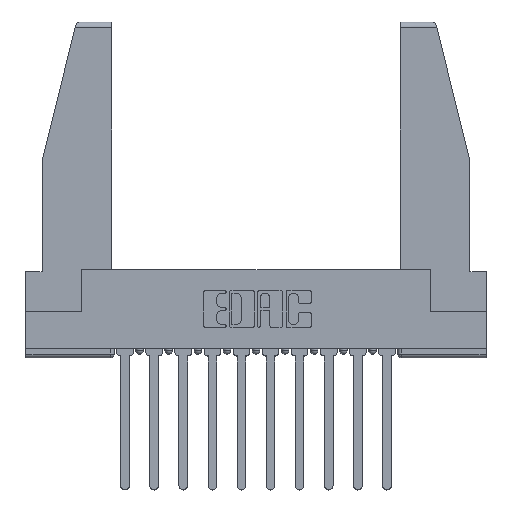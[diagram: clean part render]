
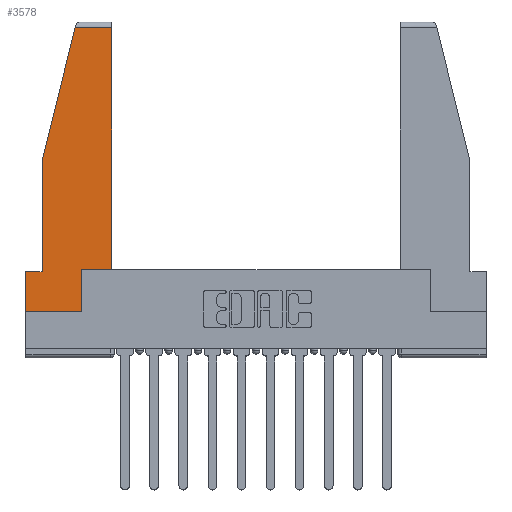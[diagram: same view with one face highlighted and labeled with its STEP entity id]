
A CAD part, top view. The second image highlights one B-rep face of the part: STEP entity #3578.
In plain terms, the highlighted planar face has unit normal (0, 0, 1).
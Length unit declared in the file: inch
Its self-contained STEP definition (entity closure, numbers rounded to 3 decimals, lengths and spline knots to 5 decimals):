
#171 = VECTOR ( 'NONE', #4945, 39.37008 ) ;
#489 = ORIENTED_EDGE ( 'NONE', *, *, #1004, .T. ) ;
#675 = LINE ( 'NONE', #2771, #14675 ) ;
#927 = FACE_OUTER_BOUND ( 'NONE', #11522, .T. ) ;
#1004 = EDGE_CURVE ( 'NONE', #10563, #9071, #10945, .T. ) ;
#1023 = CARTESIAN_POINT ( 'NONE',  ( 0.2636, 1.52, 0. ) ) ;
#1205 = EDGE_CURVE ( 'NONE', #8039, #13820, #3574, .T. ) ;
#1233 = VERTEX_POINT ( 'NONE', #8823 ) ;
#1274 = VECTOR ( 'NONE', #9186, 39.37008 ) ;
#1566 = EDGE_CURVE ( 'NONE', #1233, #8039, #10570, .T. ) ;
#1838 = DIRECTION ( 'NONE',  ( 0., 1., 0. ) ) ;
#2105 = VECTOR ( 'NONE', #6671, 39.37008 ) ;
#2409 = AXIS2_PLACEMENT_3D ( 'NONE', #7651, #11074, #8683 ) ;
#2624 = VERTEX_POINT ( 'NONE', #4546 ) ;
#2654 = ORIENTED_EDGE ( 'NONE', *, *, #11055, .T. ) ;
#2771 = CARTESIAN_POINT ( 'NONE',  ( 0., 0.21, 0. ) ) ;
#2823 = CARTESIAN_POINT ( 'NONE',  ( 0., 0.21, 0. ) ) ;
#2879 = DIRECTION ( 'NONE',  ( 0., -1., 0. ) ) ;
#3443 = EDGE_CURVE ( 'NONE', #7910, #9589, #12347, .T. ) ;
#3574 = LINE ( 'NONE', #14794, #12434 ) ;
#3578 = ADVANCED_FACE ( 'NONE', ( #927 ), #8742, .T. ) ;
#3805 = CARTESIAN_POINT ( 'NONE',  ( 0.461, 0.223, 0. ) ) ;
#4299 = VECTOR ( 'NONE', #13237, 39.37008 ) ;
#4369 = CARTESIAN_POINT ( 'NONE',  ( 0., 1.52, 0. ) ) ;
#4546 = CARTESIAN_POINT ( 'NONE',  ( 0.297, 0.223, 0. ) ) ;
#4945 = DIRECTION ( 'NONE',  ( 0., 1., 0. ) ) ;
#5190 = VECTOR ( 'NONE', #1838, 39.37008 ) ;
#5226 = CARTESIAN_POINT ( 'NONE',  ( 0.086, 0.21, 0. ) ) ;
#5296 = CARTESIAN_POINT ( 'NONE',  ( 0.297, 0., 0. ) ) ;
#5625 = VECTOR ( 'NONE', #13990, 39.37008 ) ;
#5702 = CARTESIAN_POINT ( 'NONE',  ( 0., 0., 0. ) ) ;
#6037 = CARTESIAN_POINT ( 'NONE',  ( 0.271, 1.55, 0. ) ) ;
#6671 = DIRECTION ( 'NONE',  ( 1., 0., 0. ) ) ;
#7025 = CARTESIAN_POINT ( 'NONE',  ( 0.461, 1.52, 0. ) ) ;
#7330 = CARTESIAN_POINT ( 'NONE',  ( 0.297, 0., 0. ) ) ;
#7535 = DIRECTION ( 'NONE',  ( 0., -1., 0. ) ) ;
#7651 = CARTESIAN_POINT ( 'NONE',  ( 0., 0., 0. ) ) ;
#7776 = CARTESIAN_POINT ( 'NONE',  ( 0., 0., 0. ) ) ;
#7782 = VERTEX_POINT ( 'NONE', #1023 ) ;
#7910 = VERTEX_POINT ( 'NONE', #8453 ) ;
#8039 = VERTEX_POINT ( 'NONE', #5226 ) ;
#8453 = CARTESIAN_POINT ( 'NONE',  ( 0.461, 0.223, 0. ) ) ;
#8683 = DIRECTION ( 'NONE',  ( 1., 0., 0. ) ) ;
#8742 = PLANE ( 'NONE',  #2409 ) ;
#8823 = CARTESIAN_POINT ( 'NONE',  ( 0.086, 0.8, 0. ) ) ;
#8929 = LINE ( 'NONE', #6037, #4299 ) ;
#9071 = VERTEX_POINT ( 'NONE', #7330 ) ;
#9186 = DIRECTION ( 'NONE',  ( -1., 0., 0. ) ) ;
#9356 = EDGE_CURVE ( 'NONE', #9589, #7782, #11591, .T. ) ;
#9589 = VERTEX_POINT ( 'NONE', #7025 ) ;
#9765 = ORIENTED_EDGE ( 'NONE', *, *, #9356, .T. ) ;
#9850 = LINE ( 'NONE', #5296, #5190 ) ;
#10126 = DIRECTION ( 'NONE',  ( -1., 0., 0. ) ) ;
#10563 = VERTEX_POINT ( 'NONE', #7776 ) ;
#10570 = LINE ( 'NONE', #10745, #11122 ) ;
#10745 = CARTESIAN_POINT ( 'NONE',  ( 0.086, 0.8, 0. ) ) ;
#10945 = LINE ( 'NONE', #5702, #2105 ) ;
#11055 = EDGE_CURVE ( 'NONE', #13820, #10563, #675, .T. ) ;
#11074 = DIRECTION ( 'NONE',  ( 0., 0., 1. ) ) ;
#11122 = VECTOR ( 'NONE', #7535, 39.37008 ) ;
#11522 = EDGE_LOOP ( 'NONE', ( #14370, #9765, #12956, #14327, #12271, #2654, #489, #13171, #12616 ) ) ;
#11591 = LINE ( 'NONE', #4369, #1274 ) ;
#11912 = EDGE_CURVE ( 'NONE', #2624, #7910, #15023, .T. ) ;
#12271 = ORIENTED_EDGE ( 'NONE', *, *, #1205, .T. ) ;
#12347 = LINE ( 'NONE', #3805, #171 ) ;
#12434 = VECTOR ( 'NONE', #10126, 39.37008 ) ;
#12609 = CARTESIAN_POINT ( 'NONE',  ( 0.297, 0.223, 0. ) ) ;
#12616 = ORIENTED_EDGE ( 'NONE', *, *, #11912, .T. ) ;
#12956 = ORIENTED_EDGE ( 'NONE', *, *, #13691, .T. ) ;
#13171 = ORIENTED_EDGE ( 'NONE', *, *, #14377, .T. ) ;
#13237 = DIRECTION ( 'NONE',  ( -0.239, -0.971, 0. ) ) ;
#13691 = EDGE_CURVE ( 'NONE', #7782, #1233, #8929, .T. ) ;
#13820 = VERTEX_POINT ( 'NONE', #2823 ) ;
#13990 = DIRECTION ( 'NONE',  ( 1., 0., 0. ) ) ;
#14327 = ORIENTED_EDGE ( 'NONE', *, *, #1566, .T. ) ;
#14370 = ORIENTED_EDGE ( 'NONE', *, *, #3443, .T. ) ;
#14377 = EDGE_CURVE ( 'NONE', #9071, #2624, #9850, .T. ) ;
#14675 = VECTOR ( 'NONE', #2879, 39.37008 ) ;
#14794 = CARTESIAN_POINT ( 'NONE',  ( 0., 0.21, 0. ) ) ;
#15023 = LINE ( 'NONE', #12609, #5625 ) ;
